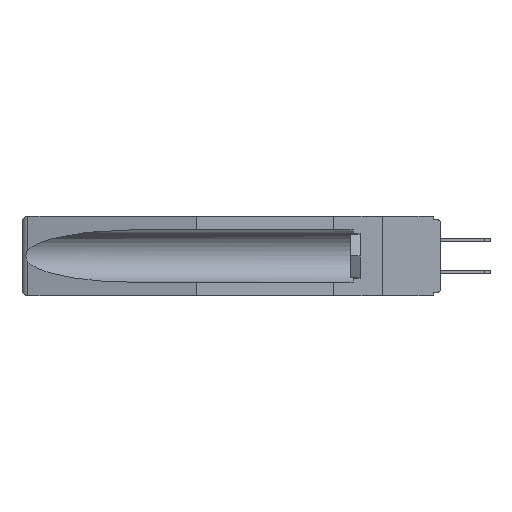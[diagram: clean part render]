
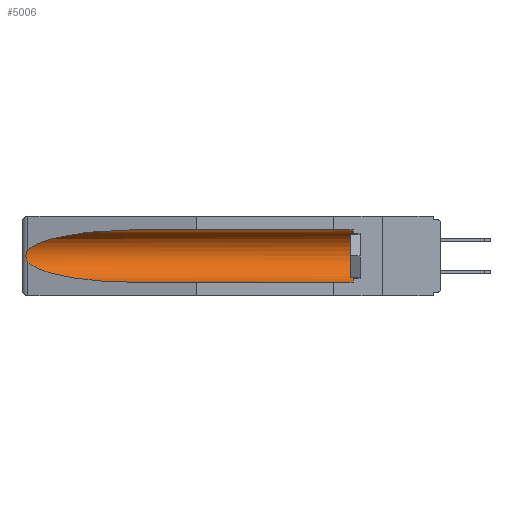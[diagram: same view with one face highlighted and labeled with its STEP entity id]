
A CAD part, left-side view. The second image highlights one B-rep face of the part: STEP entity #5006.
In plain terms, the highlighted cylindrical face has radius 2.857 mm (diameter 5.715 mm), a partial arc.
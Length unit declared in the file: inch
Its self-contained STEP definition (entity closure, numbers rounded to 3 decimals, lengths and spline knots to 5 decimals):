
#131 = AXIS2_PLACEMENT_3D ( 'NONE', #19291, #8297, #6532 ) ;
#1238 = DIRECTION ( 'NONE',  ( 0., 1., 0. ) ) ;
#1454 = CARTESIAN_POINT ( 'NONE',  ( 0.26654, 1.53092, -0.15636 ) ) ;
#2121 = CARTESIAN_POINT ( 'NONE',  ( 0.155, 1.07973, -0.284 ) ) ;
#2769 = EDGE_LOOP ( 'NONE', ( #16712, #15832, #16695, #11951, #19408, #15945 ) ) ;
#4400 = B_SPLINE_CURVE_WITH_KNOTS ( 'NONE', 3,
 ( #16109, #16283, #1454, #5186, #14552, #18209, #18038, #10904, #16781, #14710 ),
 .UNSPECIFIED., .F., .F.,
 ( 4, 2, 2, 2, 4 ),
 ( 0., 0.00029, 0.00058, 0.00087, 0.00117 ),
 .UNSPECIFIED. ) ;
#4664 = VERTEX_POINT ( 'NONE', #15429 ) ;
#4773 = CARTESIAN_POINT ( 'NONE',  ( 0.25451, 1.48313, -0.09465 ) ) ;
#4898 = CARTESIAN_POINT ( 'NONE',  ( 0.155, -0.30754, -0.1715 ) ) ;
#4992 = CARTESIAN_POINT ( 'NONE',  ( 0.155, -0.30754, -0.059 ) ) ;
#5006 = ADVANCED_FACE ( 'NONE', ( #10477 ), #21427, .F. ) ;
#5096 = VECTOR ( 'NONE', #6785, 39.37008 ) ;
#5186 = CARTESIAN_POINT ( 'NONE',  ( 0.2673, 1.5327, -0.16383 ) ) ;
#6532 = DIRECTION ( 'NONE',  ( 0., 0., 1. ) ) ;
#6771 = DIRECTION ( 'NONE',  ( 0., 0., 1. ) ) ;
#6785 = DIRECTION ( 'NONE',  ( 0., 1., 0. ) ) ;
#6876 = DIRECTION ( 'NONE',  ( 0., 1., 0. ) ) ;
#6951 =( BOUNDED_CURVE ( )  B_SPLINE_CURVE ( 3, ( #20357, #16694, #22052, #2121 ),
 .UNSPECIFIED., .F., .F. ) 
 B_SPLINE_CURVE_WITH_KNOTS ( ( 4, 4 ),
 ( 0.1948, 1.5708 ),
 .UNSPECIFIED. ) 
 CURVE ( )  GEOMETRIC_REPRESENTATION_ITEM ( )  RATIONAL_B_SPLINE_CURVE ( ( 1., 0.848, 0.848, 1. ) ) 
 REPRESENTATION_ITEM ( '' )  );
#8261 = CARTESIAN_POINT ( 'NONE',  ( 0.21114, 1.30732, -0.059 ) ) ;
#8297 = DIRECTION ( 'NONE',  ( 0., -1., 0. ) ) ;
#9110 = CARTESIAN_POINT ( 'NONE',  ( 0.155, 1.07973, -0.284 ) ) ;
#9719 = CARTESIAN_POINT ( 'NONE',  ( 0.155, 1.07973, -0.059 ) ) ;
#10477 = FACE_OUTER_BOUND ( 'NONE', #2769, .T. ) ;
#10904 = CARTESIAN_POINT ( 'NONE',  ( 0.26655, 1.53094, -0.18657 ) ) ;
#11007 = EDGE_CURVE ( 'NONE', #19360, #13924, #4400, .T. ) ;
#11854 = CARTESIAN_POINT ( 'NONE',  ( 0.26537, 1.52718, -0.14972 ) ) ;
#11951 = ORIENTED_EDGE ( 'NONE', *, *, #21136, .F. ) ;
#11978 = CARTESIAN_POINT ( 'NONE',  ( 0.155, 1.07973, -0.059 ) ) ;
#13924 = VERTEX_POINT ( 'NONE', #15326 ) ;
#14240 = EDGE_CURVE ( 'NONE', #13924, #18418, #6951, .T. ) ;
#14552 = CARTESIAN_POINT ( 'NONE',  ( 0.2675, 1.53308, -0.16763 ) ) ;
#14676 = VERTEX_POINT ( 'NONE', #19343 ) ;
#14710 = CARTESIAN_POINT ( 'NONE',  ( 0.26537, 1.52718, -0.19328 ) ) ;
#15326 = CARTESIAN_POINT ( 'NONE',  ( 0.26537, 1.52718, -0.19328 ) ) ;
#15429 = CARTESIAN_POINT ( 'NONE',  ( 0.155, 0.126, -0.284 ) ) ;
#15727 = LINE ( 'NONE', #4992, #21188 ) ;
#15832 = ORIENTED_EDGE ( 'NONE', *, *, #11007, .T. ) ;
#15945 = ORIENTED_EDGE ( 'NONE', *, *, #20482, .T. ) ;
#16109 = CARTESIAN_POINT ( 'NONE',  ( 0.26537, 1.52718, -0.14972 ) ) ;
#16283 = CARTESIAN_POINT ( 'NONE',  ( 0.26597, 1.52961, -0.15275 ) ) ;
#16350 = AXIS2_PLACEMENT_3D ( 'NONE', #4898, #1238, #6771 ) ;
#16694 = CARTESIAN_POINT ( 'NONE',  ( 0.25451, 1.48313, -0.24835 ) ) ;
#16695 = ORIENTED_EDGE ( 'NONE', *, *, #14240, .T. ) ;
#16712 = ORIENTED_EDGE ( 'NONE', *, *, #23748, .T. ) ;
#16781 = CARTESIAN_POINT ( 'NONE',  ( 0.26597, 1.5296, -0.19026 ) ) ;
#17379 = EDGE_CURVE ( 'NONE', #4664, #14676, #22680, .T. ) ;
#18038 = CARTESIAN_POINT ( 'NONE',  ( 0.2673, 1.53269, -0.17917 ) ) ;
#18209 = CARTESIAN_POINT ( 'NONE',  ( 0.2675, 1.53308, -0.17534 ) ) ;
#18418 = VERTEX_POINT ( 'NONE', #9110 ) ;
#19047 = VERTEX_POINT ( 'NONE', #9719 ) ;
#19291 = CARTESIAN_POINT ( 'NONE',  ( 0.155, 0.126, -0.1715 ) ) ;
#19343 = CARTESIAN_POINT ( 'NONE',  ( 0.155, 0.126, -0.059 ) ) ;
#19360 = VERTEX_POINT ( 'NONE', #11854 ) ;
#19408 = ORIENTED_EDGE ( 'NONE', *, *, #17379, .T. ) ;
#19768 = CARTESIAN_POINT ( 'NONE',  ( 0.155, -0.30754, -0.284 ) ) ;
#20357 = CARTESIAN_POINT ( 'NONE',  ( 0.26537, 1.52718, -0.19328 ) ) ;
#20482 = EDGE_CURVE ( 'NONE', #14676, #19047, #15727, .T. ) ;
#21136 = EDGE_CURVE ( 'NONE', #4664, #18418, #22921, .T. ) ;
#21188 = VECTOR ( 'NONE', #6876, 39.37008 ) ;
#21193 =( BOUNDED_CURVE ( )  B_SPLINE_CURVE ( 3, ( #11978, #8261, #4773, #23094 ),
 .UNSPECIFIED., .F., .F. ) 
 B_SPLINE_CURVE_WITH_KNOTS ( ( 4, 4 ),
 ( 4.71239, 6.08839 ),
 .UNSPECIFIED. ) 
 CURVE ( )  GEOMETRIC_REPRESENTATION_ITEM ( )  RATIONAL_B_SPLINE_CURVE ( ( 1., 0.848, 0.848, 1. ) ) 
 REPRESENTATION_ITEM ( '' )  );
#21427 = CYLINDRICAL_SURFACE ( 'NONE', #16350, 0.1125 ) ;
#22052 = CARTESIAN_POINT ( 'NONE',  ( 0.21114, 1.30732, -0.284 ) ) ;
#22680 = CIRCLE ( 'NONE', #131, 0.1125 ) ;
#22921 = LINE ( 'NONE', #19768, #5096 ) ;
#23094 = CARTESIAN_POINT ( 'NONE',  ( 0.26537, 1.52718, -0.14972 ) ) ;
#23748 = EDGE_CURVE ( 'NONE', #19047, #19360, #21193, .T. ) ;
